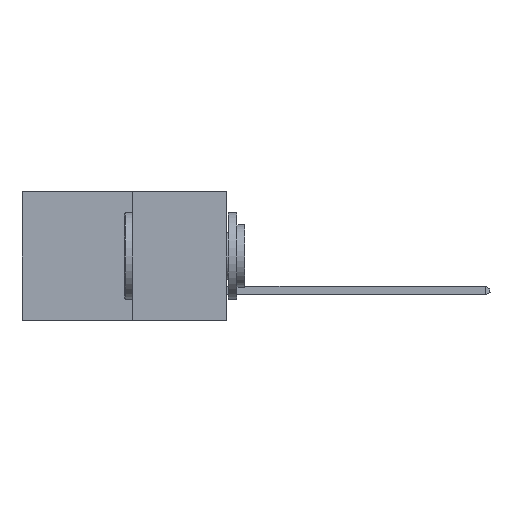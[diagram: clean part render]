
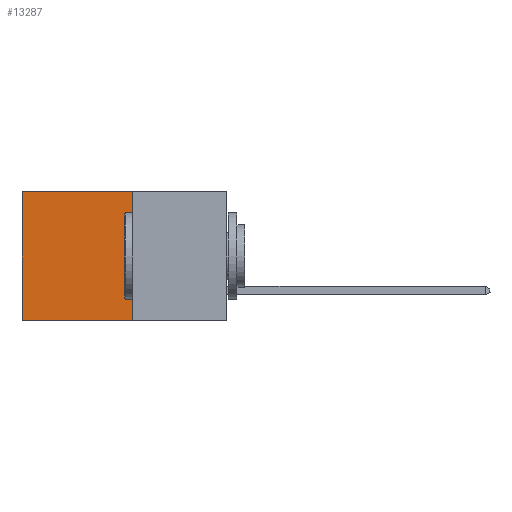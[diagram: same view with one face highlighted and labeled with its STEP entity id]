
A CAD part, left-side view. The second image highlights one B-rep face of the part: STEP entity #13287.
In plain terms, the highlighted planar face has unit normal (-1, 0, 0).
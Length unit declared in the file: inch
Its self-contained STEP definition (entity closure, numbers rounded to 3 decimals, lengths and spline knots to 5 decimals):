
#1493 = EDGE_CURVE ( 'NONE', #24319, #8968, #4855, .T. ) ;
#2744 = ORIENTED_EDGE ( 'NONE', *, *, #19609, .F. ) ;
#4371 = DIRECTION ( 'NONE',  ( 0., 0., -1. ) ) ;
#4855 = LINE ( 'NONE', #21774, #31584 ) ;
#6162 = EDGE_CURVE ( 'NONE', #6548, #24319, #8356, .T. ) ;
#6548 = VERTEX_POINT ( 'NONE', #19102 ) ;
#7002 = CARTESIAN_POINT ( 'NONE',  ( 0.277, 0.27, -0.37 ) ) ;
#7554 = EDGE_CURVE ( 'NONE', #6548, #19317, #12732, .T. ) ;
#8356 = LINE ( 'NONE', #12252, #14429 ) ;
#8481 = CARTESIAN_POINT ( 'NONE',  ( 0.277, 0.27, -0.37 ) ) ;
#8968 = VERTEX_POINT ( 'NONE', #9035 ) ;
#9035 = CARTESIAN_POINT ( 'NONE',  ( 0.277, 0.59, -0.37 ) ) ;
#9915 = EDGE_LOOP ( 'NONE', ( #18650, #2744, #25704, #20503 ) ) ;
#10473 = LINE ( 'NONE', #22508, #30252 ) ;
#11821 = DIRECTION ( 'NONE',  ( 0., 1., 0. ) ) ;
#11927 = VECTOR ( 'NONE', #19551, 39.37008 ) ;
#12252 = CARTESIAN_POINT ( 'NONE',  ( 0.277, 0.27, 0. ) ) ;
#12732 = LINE ( 'NONE', #7002, #11927 ) ;
#12776 = FACE_OUTER_BOUND ( 'NONE', #9915, .T. ) ;
#13287 = ADVANCED_FACE ( 'NONE', ( #12776 ), #32830, .F. ) ;
#14429 = VECTOR ( 'NONE', #11821, 39.37008 ) ;
#17254 = DIRECTION ( 'NONE',  ( 0., 1., 0. ) ) ;
#17316 = CARTESIAN_POINT ( 'NONE',  ( 0.277, 0.27, -0.37 ) ) ;
#18650 = ORIENTED_EDGE ( 'NONE', *, *, #1493, .T. ) ;
#19102 = CARTESIAN_POINT ( 'NONE',  ( 0.277, 0.27, 0. ) ) ;
#19317 = VERTEX_POINT ( 'NONE', #8481 ) ;
#19551 = DIRECTION ( 'NONE',  ( 0., 0., -1. ) ) ;
#19609 = EDGE_CURVE ( 'NONE', #19317, #8968, #10473, .T. ) ;
#19926 = DIRECTION ( 'NONE',  ( 1., 0., 0. ) ) ;
#20503 = ORIENTED_EDGE ( 'NONE', *, *, #6162, .T. ) ;
#21774 = CARTESIAN_POINT ( 'NONE',  ( 0.277, 0.59, -0.37 ) ) ;
#22508 = CARTESIAN_POINT ( 'NONE',  ( 0.277, 0.27, -0.37 ) ) ;
#22672 = DIRECTION ( 'NONE',  ( 0., 0., -1. ) ) ;
#23790 = CARTESIAN_POINT ( 'NONE',  ( 0.277, 0.59, 0. ) ) ;
#24319 = VERTEX_POINT ( 'NONE', #23790 ) ;
#25704 = ORIENTED_EDGE ( 'NONE', *, *, #7554, .F. ) ;
#28724 = AXIS2_PLACEMENT_3D ( 'NONE', #17316, #19926, #4371 ) ;
#30252 = VECTOR ( 'NONE', #17254, 39.37008 ) ;
#31584 = VECTOR ( 'NONE', #22672, 39.37008 ) ;
#32830 = PLANE ( 'NONE',  #28724 ) ;
